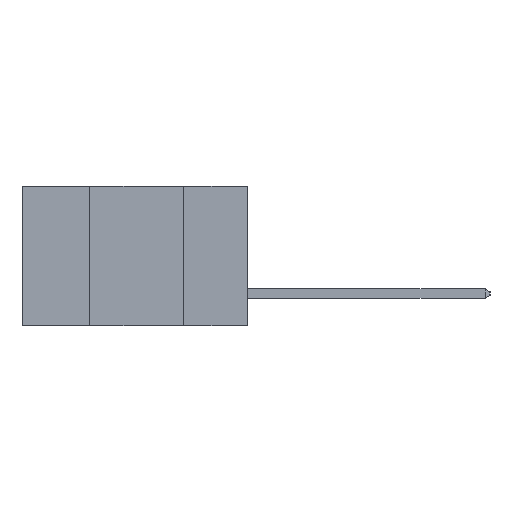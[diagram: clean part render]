
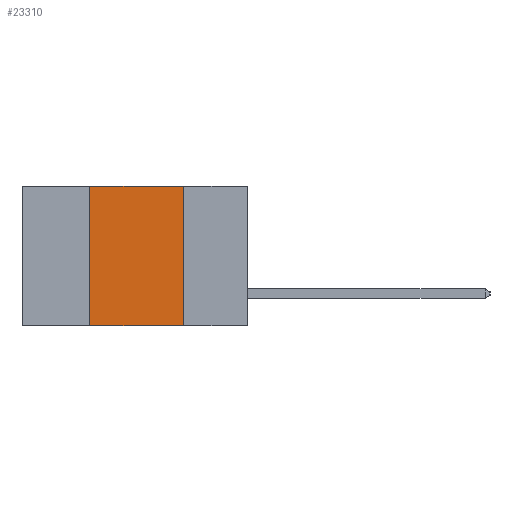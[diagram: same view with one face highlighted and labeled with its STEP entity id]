
A CAD part, left-side view. The second image highlights one B-rep face of the part: STEP entity #23310.
In plain terms, the highlighted planar face has unit normal (-1, 0, 0).
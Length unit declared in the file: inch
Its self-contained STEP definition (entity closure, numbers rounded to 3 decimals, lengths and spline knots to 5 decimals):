
#104 = LINE ( 'NONE', #20896, #26754 ) ;
#108 = EDGE_CURVE ( 'NONE', #9394, #19727, #104, .T. ) ;
#1117 = LINE ( 'NONE', #18906, #14253 ) ;
#2228 = VERTEX_POINT ( 'NONE', #32179 ) ;
#3030 = FACE_OUTER_BOUND ( 'NONE', #15220, .T. ) ;
#4988 = CARTESIAN_POINT ( 'NONE',  ( 0., 0.42, 0. ) ) ;
#6907 = DIRECTION ( 'NONE',  ( 0., 0., -1. ) ) ;
#8955 = ORIENTED_EDGE ( 'NONE', *, *, #25600, .T. ) ;
#9253 = CARTESIAN_POINT ( 'NONE',  ( 0., 0.6, 0. ) ) ;
#9394 = VERTEX_POINT ( 'NONE', #12615 ) ;
#11760 = LINE ( 'NONE', #9253, #17823 ) ;
#11901 = DIRECTION ( 'NONE',  ( 0., -1., 0. ) ) ;
#12251 = VERTEX_POINT ( 'NONE', #4988 ) ;
#12615 = CARTESIAN_POINT ( 'NONE',  ( 0., 0.17, 0. ) ) ;
#14253 = VECTOR ( 'NONE', #21478, 39.37008 ) ;
#14653 = ORIENTED_EDGE ( 'NONE', *, *, #19300, .F. ) ;
#15220 = EDGE_LOOP ( 'NONE', ( #33177, #14653, #28555, #8955 ) ) ;
#17823 = VECTOR ( 'NONE', #11901, 39.37008 ) ;
#18906 = CARTESIAN_POINT ( 'NONE',  ( 0., 0.42, 0. ) ) ;
#19300 = EDGE_CURVE ( 'NONE', #12251, #9394, #11760, .T. ) ;
#19727 = VERTEX_POINT ( 'NONE', #21351 ) ;
#19895 = CARTESIAN_POINT ( 'NONE',  ( 0., 0.6, 0. ) ) ;
#20896 = CARTESIAN_POINT ( 'NONE',  ( 0., 0.17, 0. ) ) ;
#21351 = CARTESIAN_POINT ( 'NONE',  ( 0., 0.17, -0.37 ) ) ;
#21478 = DIRECTION ( 'NONE',  ( 0., 0., 1. ) ) ;
#22338 = VECTOR ( 'NONE', #22971, 39.37008 ) ;
#22463 = DIRECTION ( 'NONE',  ( 1., 0., 0. ) ) ;
#22971 = DIRECTION ( 'NONE',  ( 0., -1., 0. ) ) ;
#23310 = ADVANCED_FACE ( 'NONE', ( #3030 ), #24913, .F. ) ;
#24913 = PLANE ( 'NONE',  #28959 ) ;
#25600 = EDGE_CURVE ( 'NONE', #2228, #19727, #29752, .T. ) ;
#26225 = DIRECTION ( 'NONE',  ( 0., 0., -1. ) ) ;
#26754 = VECTOR ( 'NONE', #26225, 39.37008 ) ;
#28555 = ORIENTED_EDGE ( 'NONE', *, *, #29946, .F. ) ;
#28959 = AXIS2_PLACEMENT_3D ( 'NONE', #19895, #22463, #6907 ) ;
#29752 = LINE ( 'NONE', #30456, #22338 ) ;
#29946 = EDGE_CURVE ( 'NONE', #2228, #12251, #1117, .T. ) ;
#30456 = CARTESIAN_POINT ( 'NONE',  ( 0., 0.6, -0.37 ) ) ;
#32179 = CARTESIAN_POINT ( 'NONE',  ( 0., 0.42, -0.37 ) ) ;
#33177 = ORIENTED_EDGE ( 'NONE', *, *, #108, .F. ) ;
